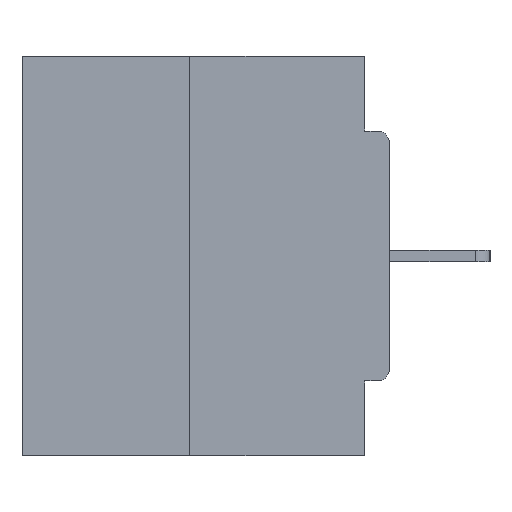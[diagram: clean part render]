
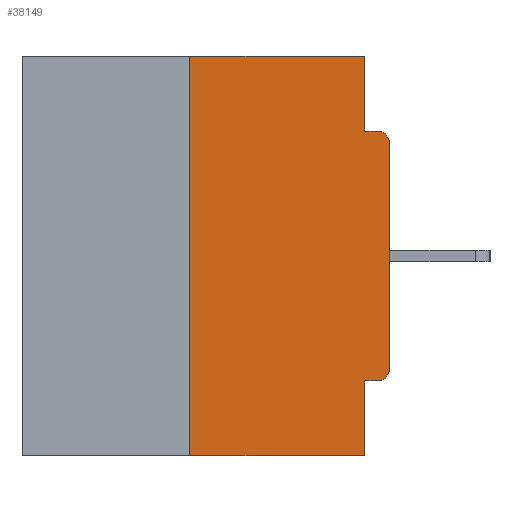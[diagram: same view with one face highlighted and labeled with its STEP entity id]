
A CAD part, left-side view. The second image highlights one B-rep face of the part: STEP entity #38149.
In plain terms, the highlighted planar face has unit normal (-1, 0, 0).
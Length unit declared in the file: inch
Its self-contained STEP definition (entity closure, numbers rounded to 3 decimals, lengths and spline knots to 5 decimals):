
#403 = CARTESIAN_POINT ( 'NONE',  ( 0., 0.015, -0.1085 ) ) ;
#705 = CARTESIAN_POINT ( 'NONE',  ( 0., 0.25, 0. ) ) ;
#1874 = ORIENTED_EDGE ( 'NONE', *, *, #31558, .F. ) ;
#2768 = DIRECTION ( 'NONE',  ( 0., 0., -1. ) ) ;
#3279 = CARTESIAN_POINT ( 'NONE',  ( 0., 0., -0.3915 ) ) ;
#3553 = DIRECTION ( 'NONE',  ( 0., 0., -1. ) ) ;
#3712 = VERTEX_POINT ( 'NONE', #32443 ) ;
#3853 = LINE ( 'NONE', #33399, #27315 ) ;
#4122 = CARTESIAN_POINT ( 'NONE',  ( 0., 0.031, 0. ) ) ;
#4276 = ORIENTED_EDGE ( 'NONE', *, *, #16749, .T. ) ;
#4962 = DIRECTION ( 'NONE',  ( 1., 0., 0. ) ) ;
#5053 = CARTESIAN_POINT ( 'NONE',  ( 0., 0.031, 0. ) ) ;
#5274 = LINE ( 'NONE', #25261, #12491 ) ;
#5346 = ORIENTED_EDGE ( 'NONE', *, *, #38208, .F. ) ;
#6218 = FACE_OUTER_BOUND ( 'NONE', #27523, .T. ) ;
#6327 = CARTESIAN_POINT ( 'NONE',  ( 0., 0.46, 0. ) ) ;
#6547 = ORIENTED_EDGE ( 'NONE', *, *, #33000, .T. ) ;
#6682 = EDGE_CURVE ( 'NONE', #18105, #27193, #15522, .T. ) ;
#6965 = AXIS2_PLACEMENT_3D ( 'NONE', #403, #21966, #3553 ) ;
#8145 = EDGE_CURVE ( 'NONE', #11586, #10926, #19673, .T. ) ;
#8218 = LINE ( 'NONE', #6327, #39507 ) ;
#9426 = DIRECTION ( 'NONE',  ( 0., -1., 0. ) ) ;
#10085 = CARTESIAN_POINT ( 'NONE',  ( 0., 0.015, -0.4065 ) ) ;
#10926 = VERTEX_POINT ( 'NONE', #39250 ) ;
#11179 = ORIENTED_EDGE ( 'NONE', *, *, #31629, .F. ) ;
#11586 = VERTEX_POINT ( 'NONE', #15778 ) ;
#12457 = VECTOR ( 'NONE', #18542, 39.37008 ) ;
#12491 = VECTOR ( 'NONE', #13127, 39.37008 ) ;
#13127 = DIRECTION ( 'NONE',  ( 0., 1., 0. ) ) ;
#14173 = PLANE ( 'NONE',  #22338 ) ;
#14508 = ORIENTED_EDGE ( 'NONE', *, *, #6682, .F. ) ;
#14836 = CARTESIAN_POINT ( 'NONE',  ( 0., 0.46, -0.5 ) ) ;
#15522 = LINE ( 'NONE', #19122, #30672 ) ;
#15761 = CARTESIAN_POINT ( 'NONE',  ( 0., 0.031, -0.4065 ) ) ;
#15778 = CARTESIAN_POINT ( 'NONE',  ( 0., 0.25, -0.5 ) ) ;
#16516 = ORIENTED_EDGE ( 'NONE', *, *, #26813, .F. ) ;
#16749 = EDGE_CURVE ( 'NONE', #29394, #16927, #20652, .T. ) ;
#16927 = VERTEX_POINT ( 'NONE', #22359 ) ;
#17789 = VECTOR ( 'NONE', #22238, 39.37008 ) ;
#17992 = CIRCLE ( 'NONE', #6965, 0.015 ) ;
#18105 = VERTEX_POINT ( 'NONE', #25448 ) ;
#18542 = DIRECTION ( 'NONE',  ( 0., 0., 1. ) ) ;
#19122 = CARTESIAN_POINT ( 'NONE',  ( 0., 0., -0.0935 ) ) ;
#19673 = LINE ( 'NONE', #705, #17789 ) ;
#20652 = LINE ( 'NONE', #27515, #12457 ) ;
#21189 = DIRECTION ( 'NONE',  ( -1., 0., 0. ) ) ;
#21387 = DIRECTION ( 'NONE',  ( 0., 0., -1. ) ) ;
#21393 = VERTEX_POINT ( 'NONE', #15761 ) ;
#21966 = DIRECTION ( 'NONE',  ( -1., 0., 0. ) ) ;
#21992 = AXIS2_PLACEMENT_3D ( 'NONE', #39196, #21189, #2768 ) ;
#22238 = DIRECTION ( 'NONE',  ( 0., 0., 1. ) ) ;
#22338 = AXIS2_PLACEMENT_3D ( 'NONE', #23326, #4962, #26380 ) ;
#22359 = CARTESIAN_POINT ( 'NONE',  ( 0., 0., -0.1085 ) ) ;
#23326 = CARTESIAN_POINT ( 'NONE',  ( 0., 0.46, 0. ) ) ;
#23599 = ORIENTED_EDGE ( 'NONE', *, *, #25254, .T. ) ;
#23977 = DIRECTION ( 'NONE',  ( 0., -1., 0. ) ) ;
#25254 = EDGE_CURVE ( 'NONE', #28413, #29394, #36172, .T. ) ;
#25261 = CARTESIAN_POINT ( 'NONE',  ( 0., 0., -0.4065 ) ) ;
#25448 = CARTESIAN_POINT ( 'NONE',  ( 0., 0.031, -0.0935 ) ) ;
#26380 = DIRECTION ( 'NONE',  ( 0., 0., -1. ) ) ;
#26813 = EDGE_CURVE ( 'NONE', #30824, #18105, #35588, .T. ) ;
#27193 = VERTEX_POINT ( 'NONE', #28604 ) ;
#27315 = VECTOR ( 'NONE', #21387, 39.37008 ) ;
#27515 = CARTESIAN_POINT ( 'NONE',  ( 0., 0., 0. ) ) ;
#27523 = EDGE_LOOP ( 'NONE', ( #11179, #28594, #6547, #1874, #5346, #23599, #4276, #28573, #14508, #16516 ) ) ;
#28413 = VERTEX_POINT ( 'NONE', #10085 ) ;
#28573 = ORIENTED_EDGE ( 'NONE', *, *, #29427, .T. ) ;
#28594 = ORIENTED_EDGE ( 'NONE', *, *, #8145, .F. ) ;
#28604 = CARTESIAN_POINT ( 'NONE',  ( 0., 0.015, -0.0935 ) ) ;
#28606 = DIRECTION ( 'NONE',  ( 0., 0., -1. ) ) ;
#28618 = VECTOR ( 'NONE', #23977, 39.37008 ) ;
#29394 = VERTEX_POINT ( 'NONE', #3279 ) ;
#29427 = EDGE_CURVE ( 'NONE', #16927, #27193, #17992, .T. ) ;
#30672 = VECTOR ( 'NONE', #37161, 39.37008 ) ;
#30824 = VERTEX_POINT ( 'NONE', #5053 ) ;
#31558 = EDGE_CURVE ( 'NONE', #21393, #3712, #3853, .T. ) ;
#31629 = EDGE_CURVE ( 'NONE', #10926, #30824, #8218, .T. ) ;
#32443 = CARTESIAN_POINT ( 'NONE',  ( 0., 0.031, -0.5 ) ) ;
#33000 = EDGE_CURVE ( 'NONE', #11586, #3712, #36601, .T. ) ;
#33399 = CARTESIAN_POINT ( 'NONE',  ( 0., 0.031, -0.5 ) ) ;
#35588 = LINE ( 'NONE', #4122, #36508 ) ;
#36172 = CIRCLE ( 'NONE', #21992, 0.015 ) ;
#36508 = VECTOR ( 'NONE', #28606, 39.37008 ) ;
#36601 = LINE ( 'NONE', #14836, #28618 ) ;
#37161 = DIRECTION ( 'NONE',  ( 0., -1., 0. ) ) ;
#38149 = ADVANCED_FACE ( 'NONE', ( #6218 ), #14173, .F. ) ;
#38208 = EDGE_CURVE ( 'NONE', #28413, #21393, #5274, .T. ) ;
#39196 = CARTESIAN_POINT ( 'NONE',  ( 0., 0.015, -0.3915 ) ) ;
#39250 = CARTESIAN_POINT ( 'NONE',  ( 0., 0.25, 0. ) ) ;
#39507 = VECTOR ( 'NONE', #9426, 39.37008 ) ;
